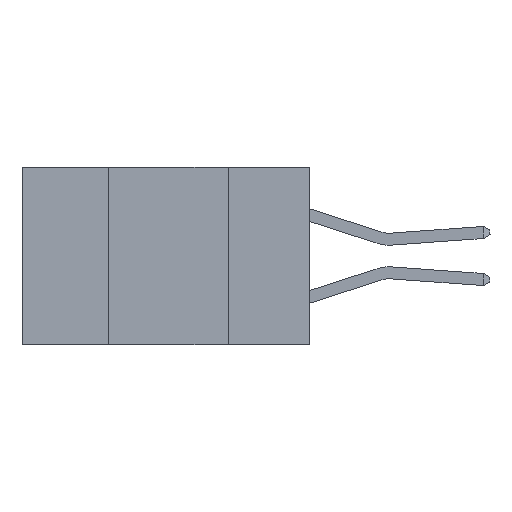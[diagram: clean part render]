
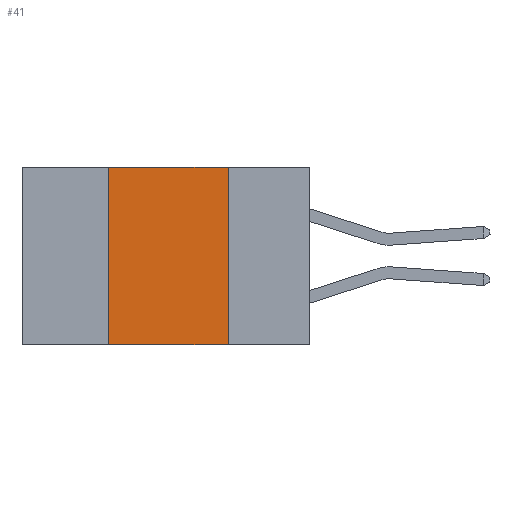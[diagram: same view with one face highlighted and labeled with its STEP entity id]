
A CAD part, left-side view. The second image highlights one B-rep face of the part: STEP entity #41.
In plain terms, the highlighted planar face has unit normal (-1, 0, 0).
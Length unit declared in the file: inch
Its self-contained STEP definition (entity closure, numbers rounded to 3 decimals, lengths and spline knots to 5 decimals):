
#41 = ADVANCED_FACE ( 'NONE', ( #9626 ), #1918, .F. ) ;
#166 = CARTESIAN_POINT ( 'NONE',  ( 0., 0.17, -0.37 ) ) ;
#204 = EDGE_CURVE ( 'NONE', #7477, #10633, #6954, .T. ) ;
#335 = DIRECTION ( 'NONE',  ( 0., 0., 1. ) ) ;
#860 = DIRECTION ( 'NONE',  ( 0., -1., 0. ) ) ;
#1566 = CARTESIAN_POINT ( 'NONE',  ( 0., 0.42, -0.37 ) ) ;
#1787 = CARTESIAN_POINT ( 'NONE',  ( 0., 0.6, 0. ) ) ;
#1853 = CARTESIAN_POINT ( 'NONE',  ( 0., 0.6, 0. ) ) ;
#1918 = PLANE ( 'NONE',  #4420 ) ;
#2208 = VECTOR ( 'NONE', #10479, 39.37008 ) ;
#2342 = LINE ( 'NONE', #9207, #12822 ) ;
#2392 = CARTESIAN_POINT ( 'NONE',  ( 0., 0.17, -0.37 ) ) ;
#2979 = VECTOR ( 'NONE', #860, 39.37008 ) ;
#3034 = DIRECTION ( 'NONE',  ( 0., 0., -1. ) ) ;
#3393 = ORIENTED_EDGE ( 'NONE', *, *, #10777, .F. ) ;
#3637 = VERTEX_POINT ( 'NONE', #166 ) ;
#3687 = CARTESIAN_POINT ( 'NONE',  ( 0., 0.42, 0. ) ) ;
#4149 = ORIENTED_EDGE ( 'NONE', *, *, #204, .F. ) ;
#4420 = AXIS2_PLACEMENT_3D ( 'NONE', #1787, #9044, #3034 ) ;
#6541 = CARTESIAN_POINT ( 'NONE',  ( 0., 0.42, -0.37 ) ) ;
#6954 = LINE ( 'NONE', #1853, #2979 ) ;
#7477 = VERTEX_POINT ( 'NONE', #3687 ) ;
#7560 = ORIENTED_EDGE ( 'NONE', *, *, #7979, .T. ) ;
#7874 = ORIENTED_EDGE ( 'NONE', *, *, #8619, .F. ) ;
#7979 = EDGE_CURVE ( 'NONE', #9439, #3637, #2342, .T. ) ;
#8286 = DIRECTION ( 'NONE',  ( 0., -1., 0. ) ) ;
#8619 = EDGE_CURVE ( 'NONE', #10633, #3637, #11329, .T. ) ;
#9044 = DIRECTION ( 'NONE',  ( 1., 0., 0. ) ) ;
#9207 = CARTESIAN_POINT ( 'NONE',  ( 0., 0.6, -0.37 ) ) ;
#9439 = VERTEX_POINT ( 'NONE', #6541 ) ;
#9607 = EDGE_LOOP ( 'NONE', ( #7874, #4149, #3393, #7560 ) ) ;
#9626 = FACE_OUTER_BOUND ( 'NONE', #9607, .T. ) ;
#10066 = LINE ( 'NONE', #1566, #12043 ) ;
#10479 = DIRECTION ( 'NONE',  ( 0., 0., -1. ) ) ;
#10633 = VERTEX_POINT ( 'NONE', #12216 ) ;
#10777 = EDGE_CURVE ( 'NONE', #9439, #7477, #10066, .T. ) ;
#11329 = LINE ( 'NONE', #2392, #2208 ) ;
#12043 = VECTOR ( 'NONE', #335, 39.37008 ) ;
#12216 = CARTESIAN_POINT ( 'NONE',  ( 0., 0.17, 0. ) ) ;
#12822 = VECTOR ( 'NONE', #8286, 39.37008 ) ;
